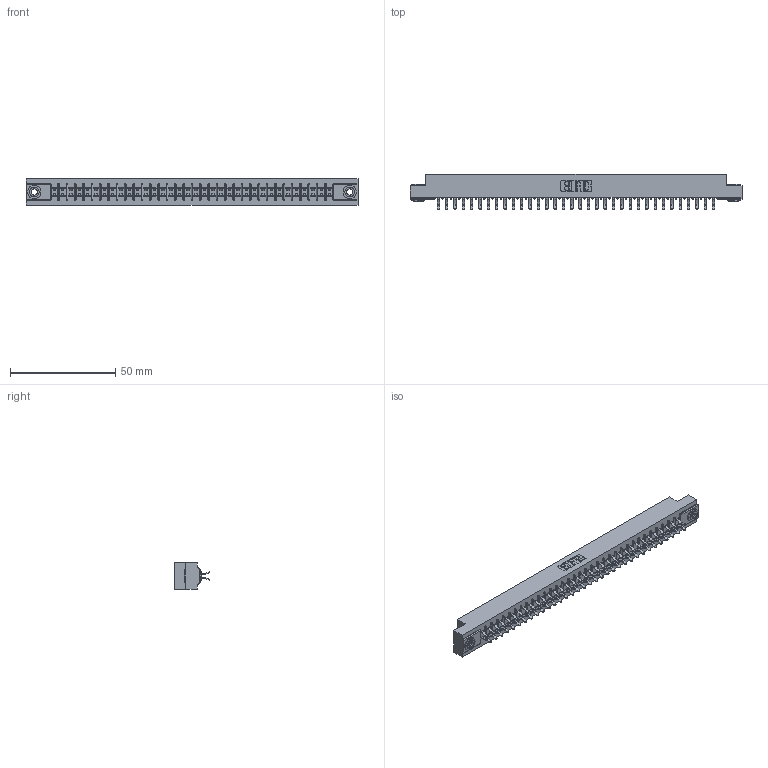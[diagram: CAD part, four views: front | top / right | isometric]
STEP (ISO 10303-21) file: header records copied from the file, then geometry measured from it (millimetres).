
FILE_DESCRIPTION (( 'STEP AP203' ), '1' );
FILE_NAME ('305-068-556-203.STEP', '2019-09-10T04:43:20', ( '' ), ( '' ), 'SwSTEP 2.0', 'SolidWorks 2016', '' );
FILE_SCHEMA (( 'CONFIG_CONTROL_DESIGN' ));
Length unit declared in the file: inch
Products named in the file (4): 305 Part_.156 Dia; 345-250-002_345-250-002-102; 305-290-001_556; 305-068-556-203
Assembly tree (71 placements, depth 2):
  305-068-556-203
    305 Part_.156 Dia
    305-290-001_556  x68
    345-250-002_345-250-002-102  x2
Bounding box: 157.73 x 16.64 x 12.7 mm (x, y, z)
Volume: 16393.4 mm3; surface area: 20955.5 mm2
Topology: 71 solids, 71 shells, 3976 faces, 11410 edges, 7420 vertices
Faces by surface type: plane 2200, cylinder 1632, sphere 136, cone 8
Entity records: 39074 total; most frequent: CARTESIAN_POINT 6449, ORIENTED_EDGE 6392, DIRECTION 6264, EDGE_CURVE 3196, LINE 2562, VECTOR 2562, VERTEX_POINT 2036, AXIS2_PLACEMENT_3D 1851
